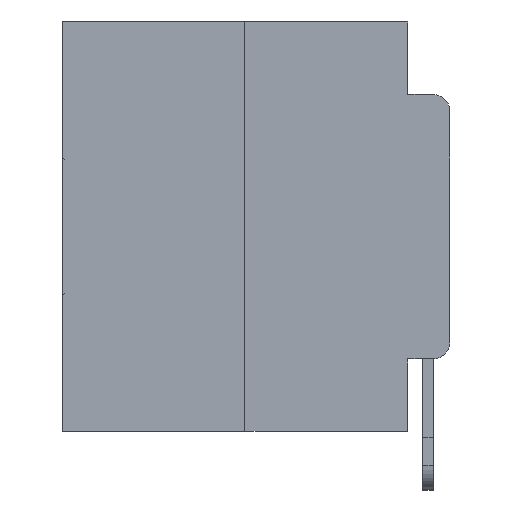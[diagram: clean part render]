
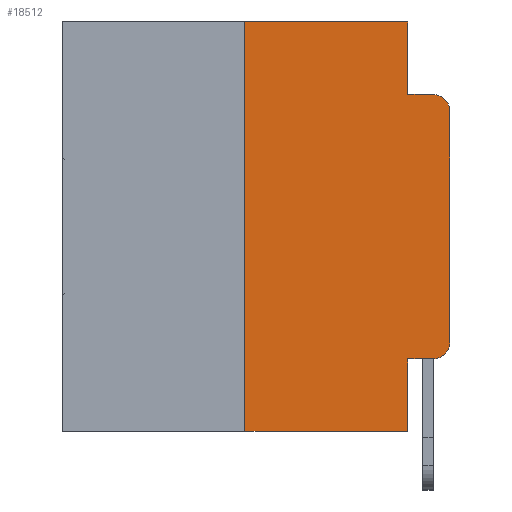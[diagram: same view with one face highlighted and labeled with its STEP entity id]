
A CAD part, left-side view. The second image highlights one B-rep face of the part: STEP entity #18512.
In plain terms, the highlighted planar face has unit normal (-1, 0, 0).
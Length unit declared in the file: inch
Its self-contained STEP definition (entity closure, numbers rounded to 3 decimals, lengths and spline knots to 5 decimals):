
#396 = CARTESIAN_POINT ( 'NONE',  ( 0., 0.473, -0.5 ) ) ;
#630 = LINE ( 'NONE', #12996, #25254 ) ;
#1012 = DIRECTION ( 'NONE',  ( 0., 0., 1. ) ) ;
#1299 = CARTESIAN_POINT ( 'NONE',  ( 0., 0.25, -0.5 ) ) ;
#1377 = CARTESIAN_POINT ( 'NONE',  ( 0., 0.051, -0.5 ) ) ;
#1424 = EDGE_CURVE ( 'NONE', #8226, #9437, #2554, .T. ) ;
#1683 = CIRCLE ( 'NONE', #19016, 0.02 ) ;
#1723 = VERTEX_POINT ( 'NONE', #10689 ) ;
#1799 = DIRECTION ( 'NONE',  ( 1., 0., 0. ) ) ;
#2202 = CARTESIAN_POINT ( 'NONE',  ( 0., 0.051, 0. ) ) ;
#2554 = LINE ( 'NONE', #18094, #20330 ) ;
#2731 = DIRECTION ( 'NONE',  ( 0., -1., 0. ) ) ;
#3215 = VECTOR ( 'NONE', #6291, 39.37008 ) ;
#4625 = CARTESIAN_POINT ( 'NONE',  ( 0., 0.02, -0.4115 ) ) ;
#5888 = AXIS2_PLACEMENT_3D ( 'NONE', #15698, #1799, #18012 ) ;
#6122 = VERTEX_POINT ( 'NONE', #2202 ) ;
#6291 = DIRECTION ( 'NONE',  ( 0., 0., -1. ) ) ;
#6646 = DIRECTION ( 'NONE',  ( -1., 0., 0. ) ) ;
#6914 = AXIS2_PLACEMENT_3D ( 'NONE', #20489, #6646, #22814 ) ;
#7005 = VERTEX_POINT ( 'NONE', #19194 ) ;
#7198 = VECTOR ( 'NONE', #13272, 39.37008 ) ;
#7565 = DIRECTION ( 'NONE',  ( -1., 0., 0. ) ) ;
#7602 = CARTESIAN_POINT ( 'NONE',  ( 0., 0.02, -0.0885 ) ) ;
#8226 = VERTEX_POINT ( 'NONE', #19317 ) ;
#8706 = EDGE_CURVE ( 'NONE', #9004, #24209, #15395, .T. ) ;
#9004 = VERTEX_POINT ( 'NONE', #1299 ) ;
#9224 = VECTOR ( 'NONE', #2731, 39.37008 ) ;
#9406 = LINE ( 'NONE', #20128, #3215 ) ;
#9437 = VERTEX_POINT ( 'NONE', #7602 ) ;
#10071 = CIRCLE ( 'NONE', #6914, 0.02 ) ;
#10689 = CARTESIAN_POINT ( 'NONE',  ( 0., 0., -0.1085 ) ) ;
#11038 = PLANE ( 'NONE',  #5888 ) ;
#11767 = EDGE_CURVE ( 'NONE', #9004, #20980, #17372, .T. ) ;
#12757 = ORIENTED_EDGE ( 'NONE', *, *, #29023, .F. ) ;
#12996 = CARTESIAN_POINT ( 'NONE',  ( 0., 0.051, -0.4115 ) ) ;
#13272 = DIRECTION ( 'NONE',  ( 0., -1., 0. ) ) ;
#13459 = EDGE_LOOP ( 'NONE', ( #27726, #27494, #14375, #19431, #26032, #17584, #25346, #12757, #19928, #15468 ) ) ;
#13551 = DIRECTION ( 'NONE',  ( 0., 0., -1. ) ) ;
#14375 = ORIENTED_EDGE ( 'NONE', *, *, #1424, .F. ) ;
#15395 = LINE ( 'NONE', #396, #9224 ) ;
#15468 = ORIENTED_EDGE ( 'NONE', *, *, #20883, .T. ) ;
#15698 = CARTESIAN_POINT ( 'NONE',  ( 0., 0.473, 0. ) ) ;
#16160 = CARTESIAN_POINT ( 'NONE',  ( 0., 0.051, -0.4115 ) ) ;
#16607 = LINE ( 'NONE', #27031, #7198 ) ;
#17204 = EDGE_CURVE ( 'NONE', #20980, #6122, #16607, .T. ) ;
#17372 = LINE ( 'NONE', #29208, #22088 ) ;
#17550 = EDGE_CURVE ( 'NONE', #1723, #9437, #1683, .T. ) ;
#17584 = ORIENTED_EDGE ( 'NONE', *, *, #11767, .F. ) ;
#17938 = VECTOR ( 'NONE', #13551, 39.37008 ) ;
#18012 = DIRECTION ( 'NONE',  ( 0., 0., -1. ) ) ;
#18094 = CARTESIAN_POINT ( 'NONE',  ( 0., 0.051, -0.0885 ) ) ;
#18512 = ADVANCED_FACE ( 'NONE', ( #23601 ), #11038, .F. ) ;
#18554 = CARTESIAN_POINT ( 'NONE',  ( 0., 0.25, 0. ) ) ;
#18784 = VECTOR ( 'NONE', #1012, 39.37008 ) ;
#19016 = AXIS2_PLACEMENT_3D ( 'NONE', #21427, #7565, #23716 ) ;
#19194 = CARTESIAN_POINT ( 'NONE',  ( 0., 0., -0.3915 ) ) ;
#19317 = CARTESIAN_POINT ( 'NONE',  ( 0., 0.051, -0.0885 ) ) ;
#19431 = ORIENTED_EDGE ( 'NONE', *, *, #20068, .F. ) ;
#19508 = LINE ( 'NONE', #28659, #18784 ) ;
#19928 = ORIENTED_EDGE ( 'NONE', *, *, #27585, .T. ) ;
#20068 = EDGE_CURVE ( 'NONE', #6122, #8226, #9406, .T. ) ;
#20098 = DIRECTION ( 'NONE',  ( 0., 0., 1. ) ) ;
#20128 = CARTESIAN_POINT ( 'NONE',  ( 0., 0.051, 0. ) ) ;
#20330 = VECTOR ( 'NONE', #27784, 39.37008 ) ;
#20489 = CARTESIAN_POINT ( 'NONE',  ( 0., 0.02, -0.3915 ) ) ;
#20883 = EDGE_CURVE ( 'NONE', #29142, #7005, #10071, .T. ) ;
#20980 = VERTEX_POINT ( 'NONE', #18554 ) ;
#21245 = EDGE_CURVE ( 'NONE', #7005, #1723, #19508, .T. ) ;
#21427 = CARTESIAN_POINT ( 'NONE',  ( 0., 0.02, -0.1085 ) ) ;
#22088 = VECTOR ( 'NONE', #20098, 39.37008 ) ;
#22814 = DIRECTION ( 'NONE',  ( 0., 0., -1. ) ) ;
#23259 = VERTEX_POINT ( 'NONE', #16160 ) ;
#23601 = FACE_OUTER_BOUND ( 'NONE', #13459, .T. ) ;
#23716 = DIRECTION ( 'NONE',  ( 0., 0., -1. ) ) ;
#24082 = LINE ( 'NONE', #27305, #17938 ) ;
#24209 = VERTEX_POINT ( 'NONE', #1377 ) ;
#24469 = DIRECTION ( 'NONE',  ( 0., -1., 0. ) ) ;
#25254 = VECTOR ( 'NONE', #24469, 39.37008 ) ;
#25346 = ORIENTED_EDGE ( 'NONE', *, *, #8706, .T. ) ;
#26032 = ORIENTED_EDGE ( 'NONE', *, *, #17204, .F. ) ;
#27031 = CARTESIAN_POINT ( 'NONE',  ( 0., 0.473, 0. ) ) ;
#27305 = CARTESIAN_POINT ( 'NONE',  ( 0., 0.051, 0. ) ) ;
#27494 = ORIENTED_EDGE ( 'NONE', *, *, #17550, .T. ) ;
#27585 = EDGE_CURVE ( 'NONE', #23259, #29142, #630, .T. ) ;
#27726 = ORIENTED_EDGE ( 'NONE', *, *, #21245, .T. ) ;
#27784 = DIRECTION ( 'NONE',  ( 0., -1., 0. ) ) ;
#28659 = CARTESIAN_POINT ( 'NONE',  ( 0., 0., 0. ) ) ;
#29023 = EDGE_CURVE ( 'NONE', #23259, #24209, #24082, .T. ) ;
#29142 = VERTEX_POINT ( 'NONE', #4625 ) ;
#29208 = CARTESIAN_POINT ( 'NONE',  ( 0., 0.25, 0. ) ) ;
